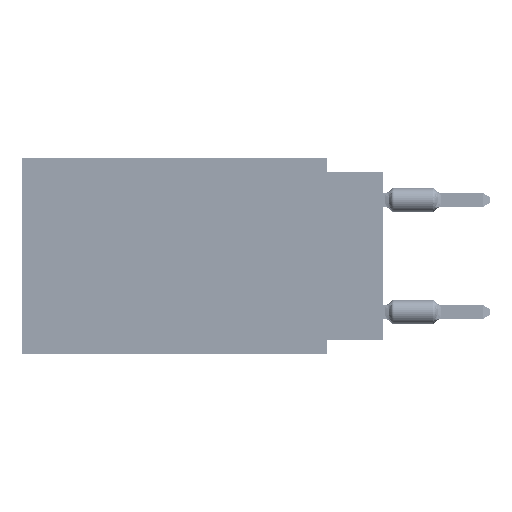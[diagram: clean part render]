
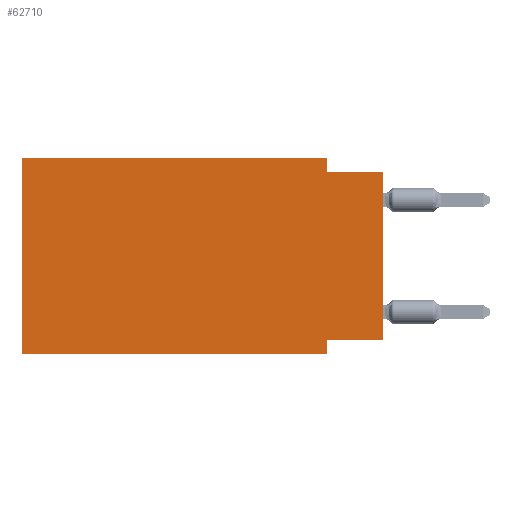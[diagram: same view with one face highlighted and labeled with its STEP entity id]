
A CAD part, left-side view. The second image highlights one B-rep face of the part: STEP entity #62710.
In plain terms, the highlighted planar face has unit normal (-1, 0, 0).
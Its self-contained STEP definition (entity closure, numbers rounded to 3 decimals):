
#171 = ORIENTED_EDGE ( 'NONE', *, *, #61118, .F. ) ;
#1784 = EDGE_CURVE ( 'NONE', #54152, #47554, #37933, .T. ) ;
#2987 = CARTESIAN_POINT ( 'NONE',  ( 0., 0., 0. ) ) ;
#3518 = CARTESIAN_POINT ( 'NONE',  ( 0., 2.54, -0.635 ) ) ;
#5776 = CARTESIAN_POINT ( 'NONE',  ( 0., 0., -8.255 ) ) ;
#5937 = DIRECTION ( 'NONE',  ( 0., -1., 0. ) ) ;
#5960 = DIRECTION ( 'NONE',  ( 0., 0., -1. ) ) ;
#8102 = ORIENTED_EDGE ( 'NONE', *, *, #44133, .F. ) ;
#8272 = DIRECTION ( 'NONE',  ( 0., 0., -1. ) ) ;
#8346 = EDGE_CURVE ( 'NONE', #27522, #18543, #10920, .T. ) ;
#10920 = LINE ( 'NONE', #5776, #54375 ) ;
#13277 = LINE ( 'NONE', #2987, #37918 ) ;
#13884 = CARTESIAN_POINT ( 'NONE',  ( 0., 2.54, -8.255 ) ) ;
#14593 = LINE ( 'NONE', #30776, #34252 ) ;
#16432 = DIRECTION ( 'NONE',  ( 0., 1., 0. ) ) ;
#17362 = VECTOR ( 'NONE', #5937, 1000. ) ;
#17369 = VECTOR ( 'NONE', #61841, 1000. ) ;
#18543 = VERTEX_POINT ( 'NONE', #13884 ) ;
#20589 = EDGE_CURVE ( 'NONE', #42711, #67283, #52662, .T. ) ;
#24285 = CARTESIAN_POINT ( 'NONE',  ( 0., 16.383, 0. ) ) ;
#24642 = VECTOR ( 'NONE', #32992, 1000. ) ;
#27522 = VERTEX_POINT ( 'NONE', #30779 ) ;
#30776 = CARTESIAN_POINT ( 'NONE',  ( 0., 16.383, 0. ) ) ;
#30779 = CARTESIAN_POINT ( 'NONE',  ( 0., 0., -8.255 ) ) ;
#31696 = ORIENTED_EDGE ( 'NONE', *, *, #69516, .T. ) ;
#32223 = CARTESIAN_POINT ( 'NONE',  ( 0., 2.54, -8.89 ) ) ;
#32992 = DIRECTION ( 'NONE',  ( 0., 0., -1. ) ) ;
#34252 = VECTOR ( 'NONE', #69319, 1000. ) ;
#35465 = FACE_OUTER_BOUND ( 'NONE', #59209, .T. ) ;
#37918 = VECTOR ( 'NONE', #63952, 1000. ) ;
#37933 = LINE ( 'NONE', #40821, #17362 ) ;
#38988 = VECTOR ( 'NONE', #68819, 1000. ) ;
#39391 = ORIENTED_EDGE ( 'NONE', *, *, #69253, .F. ) ;
#40821 = CARTESIAN_POINT ( 'NONE',  ( 0., 0., -0.635 ) ) ;
#42070 = PLANE ( 'NONE',  #69398 ) ;
#42711 = VERTEX_POINT ( 'NONE', #62354 ) ;
#44133 = EDGE_CURVE ( 'NONE', #42711, #49518, #14593, .T. ) ;
#44612 = LINE ( 'NONE', #24285, #17369 ) ;
#45094 = CARTESIAN_POINT ( 'NONE',  ( 0., 16.383, 0. ) ) ;
#46266 = EDGE_CURVE ( 'NONE', #49518, #61610, #44612, .T. ) ;
#47554 = VERTEX_POINT ( 'NONE', #55625 ) ;
#49518 = VERTEX_POINT ( 'NONE', #45094 ) ;
#49600 = VECTOR ( 'NONE', #5960, 1000. ) ;
#49986 = CARTESIAN_POINT ( 'NONE',  ( 0., 2.54, 0. ) ) ;
#52662 = LINE ( 'NONE', #62940, #38988 ) ;
#54152 = VERTEX_POINT ( 'NONE', #3518 ) ;
#54375 = VECTOR ( 'NONE', #16432, 1000. ) ;
#55625 = CARTESIAN_POINT ( 'NONE',  ( 0., 0., -0.635 ) ) ;
#57852 = CARTESIAN_POINT ( 'NONE',  ( 0., 16.383, 0. ) ) ;
#58588 = DIRECTION ( 'NONE',  ( 1., 0., 0. ) ) ;
#58599 = ORIENTED_EDGE ( 'NONE', *, *, #8346, .F. ) ;
#59209 = EDGE_LOOP ( 'NONE', ( #31696, #60232, #39391, #64756, #8102, #60939, #171, #58599 ) ) ;
#60232 = ORIENTED_EDGE ( 'NONE', *, *, #1784, .F. ) ;
#60939 = ORIENTED_EDGE ( 'NONE', *, *, #20589, .T. ) ;
#61118 = EDGE_CURVE ( 'NONE', #18543, #67283, #71885, .T. ) ;
#61420 = LINE ( 'NONE', #66939, #49600 ) ;
#61610 = VERTEX_POINT ( 'NONE', #49986 ) ;
#61841 = DIRECTION ( 'NONE',  ( 0., -1., 0. ) ) ;
#62354 = CARTESIAN_POINT ( 'NONE',  ( 0., 16.383, -8.89 ) ) ;
#62710 = ADVANCED_FACE ( 'NONE', ( #35465 ), #42070, .F. ) ;
#62940 = CARTESIAN_POINT ( 'NONE',  ( 0., 16.383, -8.89 ) ) ;
#63952 = DIRECTION ( 'NONE',  ( 0., 0., 1. ) ) ;
#64756 = ORIENTED_EDGE ( 'NONE', *, *, #46266, .F. ) ;
#66382 = CARTESIAN_POINT ( 'NONE',  ( 0., 2.54, -8.89 ) ) ;
#66939 = CARTESIAN_POINT ( 'NONE',  ( 0., 2.54, 0. ) ) ;
#67283 = VERTEX_POINT ( 'NONE', #32223 ) ;
#68819 = DIRECTION ( 'NONE',  ( 0., -1., 0. ) ) ;
#69253 = EDGE_CURVE ( 'NONE', #61610, #54152, #61420, .T. ) ;
#69319 = DIRECTION ( 'NONE',  ( 0., 0., 1. ) ) ;
#69398 = AXIS2_PLACEMENT_3D ( 'NONE', #57852, #58588, #8272 ) ;
#69516 = EDGE_CURVE ( 'NONE', #27522, #47554, #13277, .T. ) ;
#71885 = LINE ( 'NONE', #66382, #24642 ) ;
